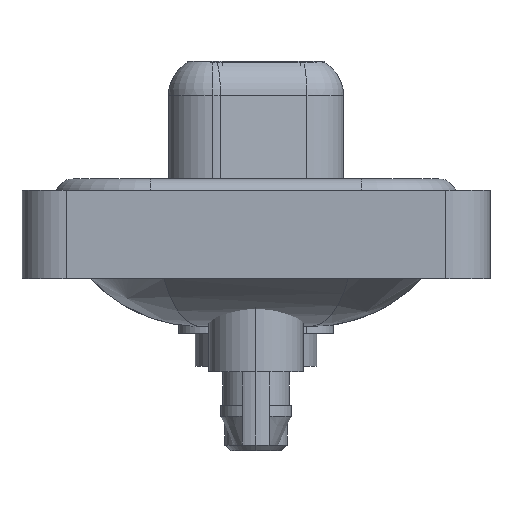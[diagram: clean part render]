
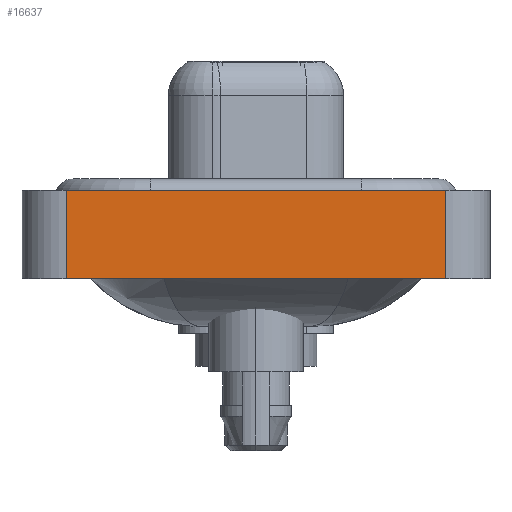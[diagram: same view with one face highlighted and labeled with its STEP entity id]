
A CAD part, left-side view. The second image highlights one B-rep face of the part: STEP entity #16637.
In plain terms, the highlighted planar face has unit normal (-1, 0, 0).
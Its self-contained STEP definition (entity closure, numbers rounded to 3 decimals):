
#147 = VECTOR ( 'NONE', #1879, 1000. ) ;
#469 = VECTOR ( 'NONE', #15618, 1000. ) ;
#648 = VERTEX_POINT ( 'NONE', #2668 ) ;
#1068 = DIRECTION ( 'NONE',  ( 0., 0., 1. ) ) ;
#1649 = ORIENTED_EDGE ( 'NONE', *, *, #11840, .F. ) ;
#1879 = DIRECTION ( 'NONE',  ( 0., 0., 1. ) ) ;
#2443 = CARTESIAN_POINT ( 'NONE',  ( -7.3, -8.55, -3.6 ) ) ;
#2596 = ORIENTED_EDGE ( 'NONE', *, *, #3213, .F. ) ;
#2668 = CARTESIAN_POINT ( 'NONE',  ( -7.3, 8.55, -3.6 ) ) ;
#3213 = EDGE_CURVE ( 'NONE', #17902, #15387, #6427, .T. ) ;
#3751 = ORIENTED_EDGE ( 'NONE', *, *, #15824, .T. ) ;
#4042 = DIRECTION ( 'NONE',  ( 0., 0., 1. ) ) ;
#4667 = CARTESIAN_POINT ( 'NONE',  ( -7.3, 8.55, -3.6 ) ) ;
#5934 = CARTESIAN_POINT ( 'NONE',  ( -7.3, -8.55, -3.6 ) ) ;
#6185 = VERTEX_POINT ( 'NONE', #15223 ) ;
#6427 = LINE ( 'NONE', #16193, #8743 ) ;
#6791 = CARTESIAN_POINT ( 'NONE',  ( -7.3, -8.55, -3.6 ) ) ;
#7235 = LINE ( 'NONE', #4667, #147 ) ;
#7811 = LINE ( 'NONE', #6791, #12776 ) ;
#8054 = DIRECTION ( 'NONE',  ( -1., 0., 0. ) ) ;
#8743 = VECTOR ( 'NONE', #9093, 1000. ) ;
#9093 = DIRECTION ( 'NONE',  ( 0., -1., 0. ) ) ;
#9424 = FACE_OUTER_BOUND ( 'NONE', #10413, .T. ) ;
#9748 = ORIENTED_EDGE ( 'NONE', *, *, #17056, .T. ) ;
#9865 = CARTESIAN_POINT ( 'NONE',  ( -7.3, 8.55, 0.4 ) ) ;
#10039 = LINE ( 'NONE', #5934, #469 ) ;
#10413 = EDGE_LOOP ( 'NONE', ( #9748, #2596, #1649, #3751 ) ) ;
#11840 = EDGE_CURVE ( 'NONE', #648, #17902, #7235, .T. ) ;
#12776 = VECTOR ( 'NONE', #4042, 1000. ) ;
#14992 = PLANE ( 'NONE',  #16533 ) ;
#15223 = CARTESIAN_POINT ( 'NONE',  ( -7.3, -8.55, -3.6 ) ) ;
#15387 = VERTEX_POINT ( 'NONE', #15741 ) ;
#15618 = DIRECTION ( 'NONE',  ( 0., -1., 0. ) ) ;
#15741 = CARTESIAN_POINT ( 'NONE',  ( -7.3, -8.55, 0.4 ) ) ;
#15824 = EDGE_CURVE ( 'NONE', #648, #6185, #10039, .T. ) ;
#16193 = CARTESIAN_POINT ( 'NONE',  ( -7.3, -8.55, 0.4 ) ) ;
#16533 = AXIS2_PLACEMENT_3D ( 'NONE', #2443, #8054, #1068 ) ;
#16637 = ADVANCED_FACE ( 'NONE', ( #9424 ), #14992, .T. ) ;
#17056 = EDGE_CURVE ( 'NONE', #6185, #15387, #7811, .T. ) ;
#17902 = VERTEX_POINT ( 'NONE', #9865 ) ;
